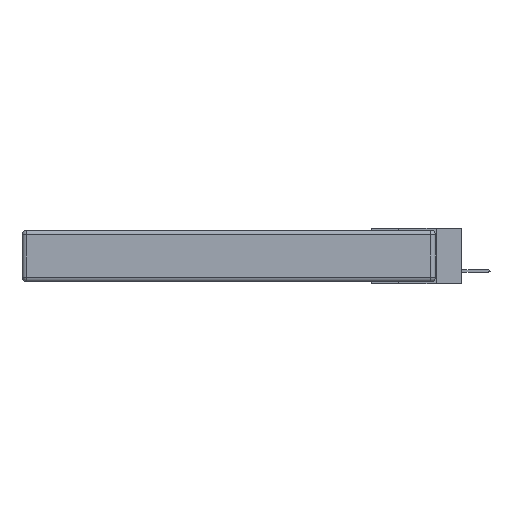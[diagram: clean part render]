
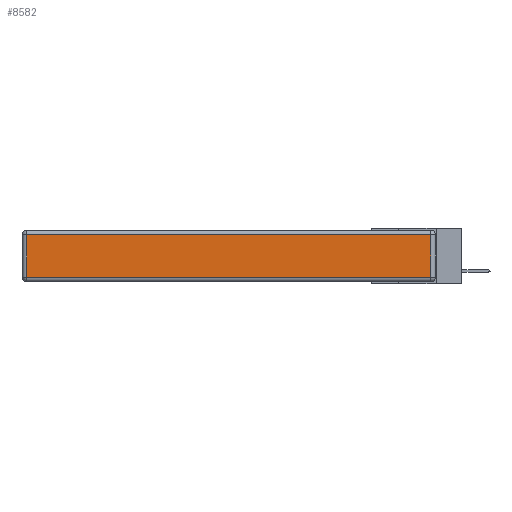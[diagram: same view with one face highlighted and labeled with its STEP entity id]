
A CAD part, left-side view. The second image highlights one B-rep face of the part: STEP entity #8582.
In plain terms, the highlighted planar face has unit normal (-1, 0, 0).
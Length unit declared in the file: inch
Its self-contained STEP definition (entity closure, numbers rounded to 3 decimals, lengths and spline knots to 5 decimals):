
#33 = DIRECTION ( 'NONE',  ( 0., 0., -1. ) ) ;
#572 = CARTESIAN_POINT ( 'NONE',  ( 0., 0.03, -0.343 ) ) ;
#993 = LINE ( 'NONE', #572, #2267 ) ;
#1787 = CARTESIAN_POINT ( 'NONE',  ( 0., 0.03, -0.313 ) ) ;
#1870 = AXIS2_PLACEMENT_3D ( 'NONE', #6716, #3302, #4524 ) ;
#2267 = VECTOR ( 'NONE', #10935, 39.37008 ) ;
#2677 = ORIENTED_EDGE ( 'NONE', *, *, #4523, .T. ) ;
#2997 = CARTESIAN_POINT ( 'NONE',  ( 0., 0., -0.313 ) ) ;
#3012 = CARTESIAN_POINT ( 'NONE',  ( 0., 0.03, -0.03 ) ) ;
#3165 = PLANE ( 'NONE',  #1870 ) ;
#3173 = EDGE_CURVE ( 'NONE', #14380, #5270, #10229, .T. ) ;
#3302 = DIRECTION ( 'NONE',  ( -1., 0., 0. ) ) ;
#3956 = ORIENTED_EDGE ( 'NONE', *, *, #10171, .T. ) ;
#4042 = LINE ( 'NONE', #2997, #7765 ) ;
#4523 = EDGE_CURVE ( 'NONE', #7280, #9441, #993, .T. ) ;
#4524 = DIRECTION ( 'NONE',  ( 0., 0., 1. ) ) ;
#4629 = FACE_OUTER_BOUND ( 'NONE', #14695, .T. ) ;
#5270 = VERTEX_POINT ( 'NONE', #8144 ) ;
#6716 = CARTESIAN_POINT ( 'NONE',  ( 0., 0., -0.343 ) ) ;
#6826 = DIRECTION ( 'NONE',  ( 0., -1., 0. ) ) ;
#7257 = ORIENTED_EDGE ( 'NONE', *, *, #3173, .T. ) ;
#7280 = VERTEX_POINT ( 'NONE', #1787 ) ;
#7656 = ORIENTED_EDGE ( 'NONE', *, *, #14264, .T. ) ;
#7765 = VECTOR ( 'NONE', #6826, 39.37008 ) ;
#7838 = VECTOR ( 'NONE', #13726, 39.37008 ) ;
#7862 = CARTESIAN_POINT ( 'NONE',  ( 0., 2.75, -0.03 ) ) ;
#8144 = CARTESIAN_POINT ( 'NONE',  ( 0., 2.72, -0.313 ) ) ;
#8205 = LINE ( 'NONE', #7862, #7838 ) ;
#8405 = CARTESIAN_POINT ( 'NONE',  ( 0., 2.72, -0.343 ) ) ;
#8582 = ADVANCED_FACE ( 'NONE', ( #4629 ), #3165, .T. ) ;
#9441 = VERTEX_POINT ( 'NONE', #3012 ) ;
#9694 = VECTOR ( 'NONE', #33, 39.37008 ) ;
#10171 = EDGE_CURVE ( 'NONE', #5270, #7280, #4042, .T. ) ;
#10229 = LINE ( 'NONE', #8405, #9694 ) ;
#10935 = DIRECTION ( 'NONE',  ( 0., 0., 1. ) ) ;
#13726 = DIRECTION ( 'NONE',  ( 0., 1., 0. ) ) ;
#14264 = EDGE_CURVE ( 'NONE', #9441, #14380, #8205, .T. ) ;
#14380 = VERTEX_POINT ( 'NONE', #14849 ) ;
#14695 = EDGE_LOOP ( 'NONE', ( #3956, #2677, #7656, #7257 ) ) ;
#14849 = CARTESIAN_POINT ( 'NONE',  ( 0., 2.72, -0.03 ) ) ;
